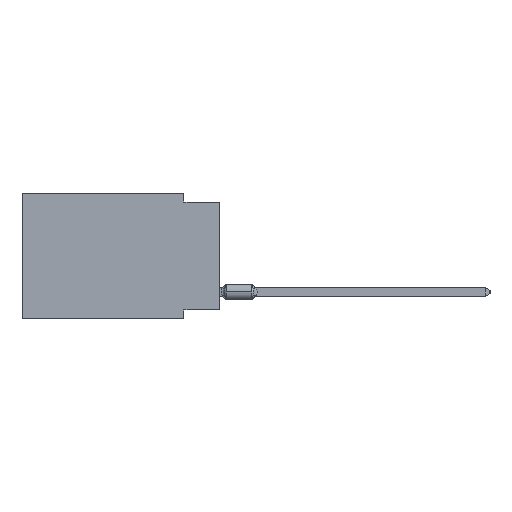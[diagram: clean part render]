
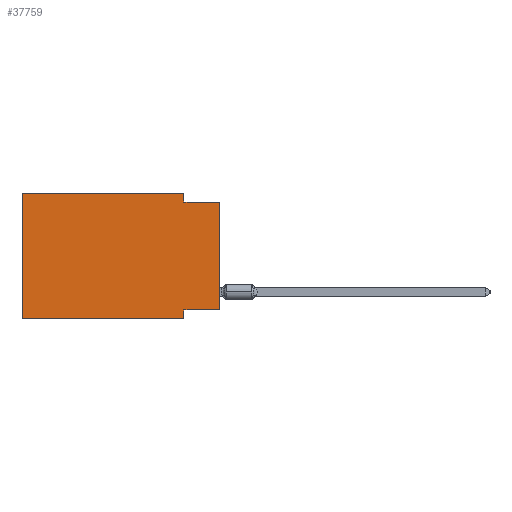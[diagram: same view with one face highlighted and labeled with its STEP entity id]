
A CAD part, left-side view. The second image highlights one B-rep face of the part: STEP entity #37759.
In plain terms, the highlighted planar face has unit normal (-1, 0, 0).
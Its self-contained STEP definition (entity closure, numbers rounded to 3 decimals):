
#1978 = VECTOR ( 'NONE', #17087, 1000. ) ;
#3123 = VERTEX_POINT ( 'NONE', #73361 ) ;
#5701 = EDGE_LOOP ( 'NONE', ( #77329, #59581, #40197, #32272, #34245, #69721, #71614, #42641 ) ) ;
#6233 = DIRECTION ( 'NONE',  ( 0., 1., 0. ) ) ;
#8802 = CARTESIAN_POINT ( 'NONE',  ( 0., 13.97, -8.89 ) ) ;
#10365 = CARTESIAN_POINT ( 'NONE',  ( 0., 2.54, -0.635 ) ) ;
#11581 = CARTESIAN_POINT ( 'NONE',  ( 0., 0., 0. ) ) ;
#12340 = EDGE_CURVE ( 'NONE', #36194, #33180, #72045, .T. ) ;
#12686 = VECTOR ( 'NONE', #58500, 1000. ) ;
#13228 = LINE ( 'NONE', #61723, #31238 ) ;
#14706 = LINE ( 'NONE', #39362, #55029 ) ;
#15540 = EDGE_CURVE ( 'NONE', #26710, #76523, #14706, .T. ) ;
#16284 = CARTESIAN_POINT ( 'NONE',  ( 0., 13.97, 0. ) ) ;
#17087 = DIRECTION ( 'NONE',  ( 0., -1., 0. ) ) ;
#17228 = DIRECTION ( 'NONE',  ( 0., 0., -1. ) ) ;
#17625 = FACE_OUTER_BOUND ( 'NONE', #5701, .T. ) ;
#19038 = EDGE_CURVE ( 'NONE', #30461, #36194, #45301, .T. ) ;
#20524 = VERTEX_POINT ( 'NONE', #26226 ) ;
#24306 = VERTEX_POINT ( 'NONE', #42696 ) ;
#26226 = CARTESIAN_POINT ( 'NONE',  ( 0., 2.54, -8.255 ) ) ;
#26710 = VERTEX_POINT ( 'NONE', #8802 ) ;
#26946 = EDGE_CURVE ( 'NONE', #3123, #33180, #63189, .T. ) ;
#27383 = CARTESIAN_POINT ( 'NONE',  ( 0., 2.54, -8.89 ) ) ;
#27937 = VECTOR ( 'NONE', #30182, 1000. ) ;
#29691 = LINE ( 'NONE', #54338, #76880 ) ;
#29738 = DIRECTION ( 'NONE',  ( 1., 0., 0. ) ) ;
#30182 = DIRECTION ( 'NONE',  ( 0., 0., 1. ) ) ;
#30461 = VERTEX_POINT ( 'NONE', #42282 ) ;
#31238 = VECTOR ( 'NONE', #62124, 1000. ) ;
#32272 = ORIENTED_EDGE ( 'NONE', *, *, #61914, .F. ) ;
#33180 = VERTEX_POINT ( 'NONE', #55021 ) ;
#33249 = CARTESIAN_POINT ( 'NONE',  ( 0., 13.97, 0. ) ) ;
#33651 = DIRECTION ( 'NONE',  ( 0., -1., 0. ) ) ;
#34245 = ORIENTED_EDGE ( 'NONE', *, *, #15540, .F. ) ;
#36194 = VERTEX_POINT ( 'NONE', #10365 ) ;
#37759 = ADVANCED_FACE ( 'NONE', ( #17625 ), #78239, .F. ) ;
#39362 = CARTESIAN_POINT ( 'NONE',  ( 0., 13.97, 0. ) ) ;
#39883 = VECTOR ( 'NONE', #33651, 1000. ) ;
#40197 = ORIENTED_EDGE ( 'NONE', *, *, #19038, .F. ) ;
#42282 = CARTESIAN_POINT ( 'NONE',  ( 0., 2.54, 0. ) ) ;
#42641 = ORIENTED_EDGE ( 'NONE', *, *, #71308, .F. ) ;
#42696 = CARTESIAN_POINT ( 'NONE',  ( 0., 2.54, -8.89 ) ) ;
#45301 = LINE ( 'NONE', #77999, #58260 ) ;
#47922 = CARTESIAN_POINT ( 'NONE',  ( 0., 13.97, 0. ) ) ;
#54338 = CARTESIAN_POINT ( 'NONE',  ( 0., 0., -8.255 ) ) ;
#55021 = CARTESIAN_POINT ( 'NONE',  ( 0., 0., -0.635 ) ) ;
#55029 = VECTOR ( 'NONE', #76542, 1000. ) ;
#58260 = VECTOR ( 'NONE', #71135, 1000. ) ;
#58500 = DIRECTION ( 'NONE',  ( 0., 0., -1. ) ) ;
#59581 = ORIENTED_EDGE ( 'NONE', *, *, #12340, .F. ) ;
#61723 = CARTESIAN_POINT ( 'NONE',  ( 0., 13.97, -8.89 ) ) ;
#61914 = EDGE_CURVE ( 'NONE', #76523, #30461, #77272, .T. ) ;
#62124 = DIRECTION ( 'NONE',  ( 0., -1., 0. ) ) ;
#62839 = EDGE_CURVE ( 'NONE', #20524, #24306, #70217, .T. ) ;
#63189 = LINE ( 'NONE', #11581, #27937 ) ;
#65974 = CARTESIAN_POINT ( 'NONE',  ( 0., 0., -0.635 ) ) ;
#66706 = AXIS2_PLACEMENT_3D ( 'NONE', #47922, #29738, #17228 ) ;
#69721 = ORIENTED_EDGE ( 'NONE', *, *, #70061, .T. ) ;
#70061 = EDGE_CURVE ( 'NONE', #26710, #24306, #13228, .T. ) ;
#70217 = LINE ( 'NONE', #27383, #12686 ) ;
#71135 = DIRECTION ( 'NONE',  ( 0., 0., -1. ) ) ;
#71308 = EDGE_CURVE ( 'NONE', #3123, #20524, #29691, .T. ) ;
#71614 = ORIENTED_EDGE ( 'NONE', *, *, #62839, .F. ) ;
#72045 = LINE ( 'NONE', #65974, #1978 ) ;
#73361 = CARTESIAN_POINT ( 'NONE',  ( 0., 0., -8.255 ) ) ;
#76523 = VERTEX_POINT ( 'NONE', #16284 ) ;
#76542 = DIRECTION ( 'NONE',  ( 0., 0., 1. ) ) ;
#76880 = VECTOR ( 'NONE', #6233, 1000. ) ;
#77272 = LINE ( 'NONE', #33249, #39883 ) ;
#77329 = ORIENTED_EDGE ( 'NONE', *, *, #26946, .T. ) ;
#77999 = CARTESIAN_POINT ( 'NONE',  ( 0., 2.54, 0. ) ) ;
#78239 = PLANE ( 'NONE',  #66706 ) ;
